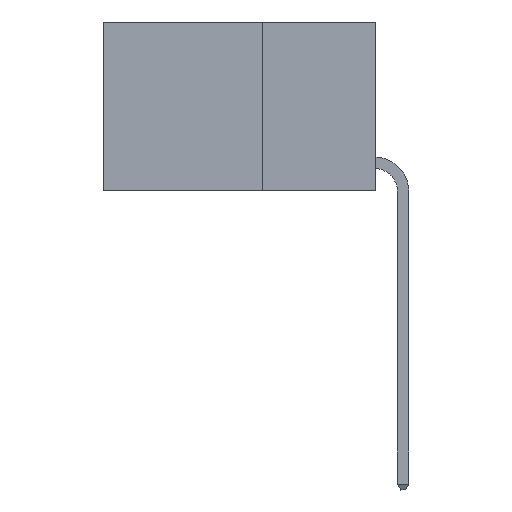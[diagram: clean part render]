
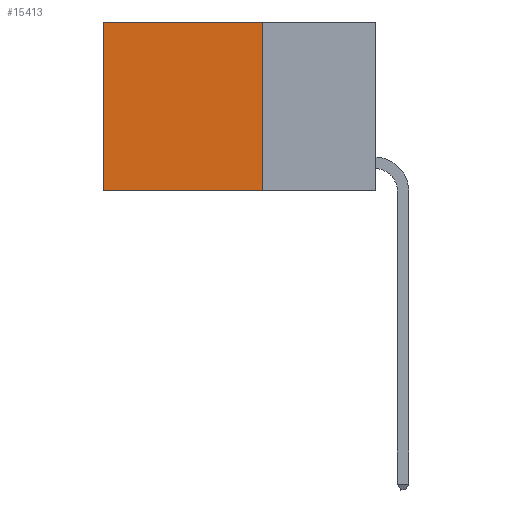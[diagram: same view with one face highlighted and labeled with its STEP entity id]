
A CAD part, left-side view. The second image highlights one B-rep face of the part: STEP entity #15413.
In plain terms, the highlighted planar face has unit normal (-1, 0, 0).
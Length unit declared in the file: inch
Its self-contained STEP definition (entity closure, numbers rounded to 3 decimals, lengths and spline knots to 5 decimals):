
#1192 = VERTEX_POINT ( 'NONE', #2323 ) ;
#1494 = LINE ( 'NONE', #15749, #8015 ) ;
#2018 = VERTEX_POINT ( 'NONE', #14805 ) ;
#2083 = VERTEX_POINT ( 'NONE', #6191 ) ;
#2321 = CARTESIAN_POINT ( 'NONE',  ( 0.2625, 0.25, 0. ) ) ;
#2323 = CARTESIAN_POINT ( 'NONE',  ( 0.2625, 0.25, 0. ) ) ;
#2539 = ORIENTED_EDGE ( 'NONE', *, *, #6390, .F. ) ;
#2750 = CARTESIAN_POINT ( 'NONE',  ( 0.2625, 0.25, 0. ) ) ;
#3096 = DIRECTION ( 'NONE',  ( 0., 1., 0. ) ) ;
#4891 = CARTESIAN_POINT ( 'NONE',  ( 0.2625, 0.6, 0. ) ) ;
#5178 = DIRECTION ( 'NONE',  ( 1., 0., 0. ) ) ;
#5193 = VECTOR ( 'NONE', #14904, 39.37008 ) ;
#6191 = CARTESIAN_POINT ( 'NONE',  ( 0.2625, 0.6, -0.37 ) ) ;
#6390 = EDGE_CURVE ( 'NONE', #1192, #2018, #16144, .T. ) ;
#6451 = EDGE_LOOP ( 'NONE', ( #8840, #8597, #2539, #15461 ) ) ;
#7021 = DIRECTION ( 'NONE',  ( 0., 1., 0. ) ) ;
#7122 = VERTEX_POINT ( 'NONE', #13862 ) ;
#7622 = PLANE ( 'NONE',  #14527 ) ;
#8015 = VECTOR ( 'NONE', #7021, 39.37008 ) ;
#8192 = VECTOR ( 'NONE', #3096, 39.37008 ) ;
#8597 = ORIENTED_EDGE ( 'NONE', *, *, #13714, .F. ) ;
#8607 = LINE ( 'NONE', #11771, #8192 ) ;
#8840 = ORIENTED_EDGE ( 'NONE', *, *, #9288, .T. ) ;
#8889 = LINE ( 'NONE', #4891, #5193 ) ;
#9288 = EDGE_CURVE ( 'NONE', #7122, #2083, #8889, .T. ) ;
#9558 = VECTOR ( 'NONE', #9728, 39.37008 ) ;
#9728 = DIRECTION ( 'NONE',  ( 0., 0., -1. ) ) ;
#11771 = CARTESIAN_POINT ( 'NONE',  ( 0.2625, 0.25, -0.37 ) ) ;
#13059 = FACE_OUTER_BOUND ( 'NONE', #6451, .T. ) ;
#13160 = EDGE_CURVE ( 'NONE', #1192, #7122, #1494, .T. ) ;
#13714 = EDGE_CURVE ( 'NONE', #2018, #2083, #8607, .T. ) ;
#13862 = CARTESIAN_POINT ( 'NONE',  ( 0.2625, 0.6, 0. ) ) ;
#13923 = DIRECTION ( 'NONE',  ( 0., 0., -1. ) ) ;
#14527 = AXIS2_PLACEMENT_3D ( 'NONE', #2750, #5178, #13923 ) ;
#14805 = CARTESIAN_POINT ( 'NONE',  ( 0.2625, 0.25, -0.37 ) ) ;
#14904 = DIRECTION ( 'NONE',  ( 0., 0., -1. ) ) ;
#15413 = ADVANCED_FACE ( 'NONE', ( #13059 ), #7622, .F. ) ;
#15461 = ORIENTED_EDGE ( 'NONE', *, *, #13160, .T. ) ;
#15749 = CARTESIAN_POINT ( 'NONE',  ( 0.2625, 0.25, 0. ) ) ;
#16144 = LINE ( 'NONE', #2321, #9558 ) ;
